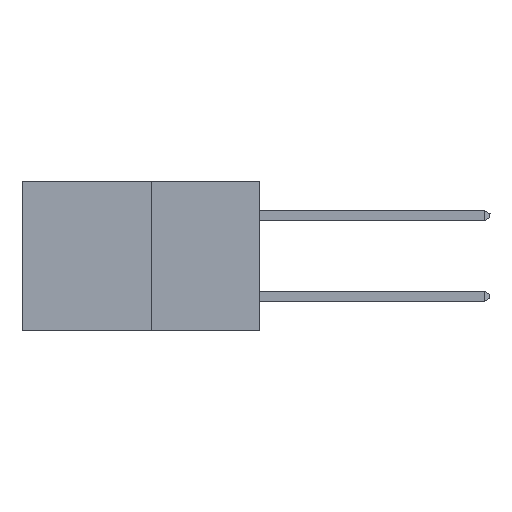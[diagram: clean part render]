
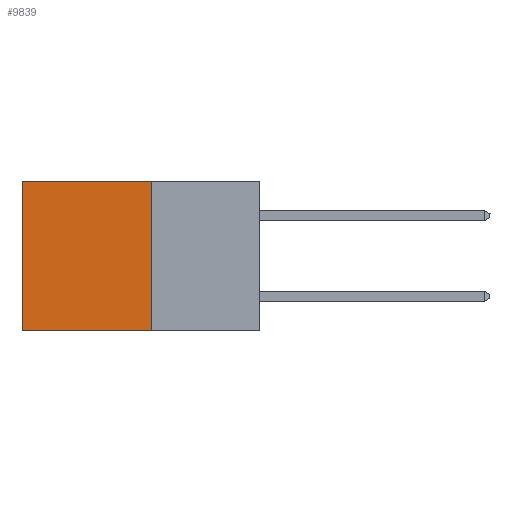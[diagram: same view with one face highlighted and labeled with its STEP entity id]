
A CAD part, left-side view. The second image highlights one B-rep face of the part: STEP entity #9839.
In plain terms, the highlighted planar face has unit normal (-1, 0, 0).
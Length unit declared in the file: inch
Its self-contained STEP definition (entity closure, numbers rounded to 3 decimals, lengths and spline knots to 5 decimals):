
#559 = VERTEX_POINT ( 'NONE', #7490 ) ;
#1075 = EDGE_CURVE ( 'NONE', #15030, #559, #17477, .T. ) ;
#1089 = VECTOR ( 'NONE', #19593, 39.37008 ) ;
#2191 = CARTESIAN_POINT ( 'NONE',  ( 0.277, 0.27, -0.37 ) ) ;
#3809 = DIRECTION ( 'NONE',  ( 0., 0., -1. ) ) ;
#5246 = ORIENTED_EDGE ( 'NONE', *, *, #15744, .T. ) ;
#5255 = DIRECTION ( 'NONE',  ( 0., 1., 0. ) ) ;
#5780 = DIRECTION ( 'NONE',  ( 0., 0., -1. ) ) ;
#6811 = LINE ( 'NONE', #18288, #15127 ) ;
#7490 = CARTESIAN_POINT ( 'NONE',  ( 0.277, 0.59, -0.37 ) ) ;
#9238 = EDGE_CURVE ( 'NONE', #15883, #559, #13239, .T. ) ;
#9664 = VECTOR ( 'NONE', #17323, 39.37008 ) ;
#9839 = ADVANCED_FACE ( 'NONE', ( #18073 ), #17810, .F. ) ;
#10019 = EDGE_CURVE ( 'NONE', #14950, #15030, #6811, .T. ) ;
#10610 = ORIENTED_EDGE ( 'NONE', *, *, #1075, .F. ) ;
#10669 = CARTESIAN_POINT ( 'NONE',  ( 0.277, 0.27, 0. ) ) ;
#11097 = ORIENTED_EDGE ( 'NONE', *, *, #10019, .F. ) ;
#11840 = ORIENTED_EDGE ( 'NONE', *, *, #9238, .T. ) ;
#13207 = DIRECTION ( 'NONE',  ( 1., 0., 0. ) ) ;
#13239 = LINE ( 'NONE', #18043, #1089 ) ;
#13891 = LINE ( 'NONE', #14625, #18014 ) ;
#13965 = CARTESIAN_POINT ( 'NONE',  ( 0.277, 0.27, -0.37 ) ) ;
#14625 = CARTESIAN_POINT ( 'NONE',  ( 0.277, 0.27, 0. ) ) ;
#14950 = VERTEX_POINT ( 'NONE', #10669 ) ;
#15030 = VERTEX_POINT ( 'NONE', #13965 ) ;
#15127 = VECTOR ( 'NONE', #5780, 39.37008 ) ;
#15744 = EDGE_CURVE ( 'NONE', #14950, #15883, #13891, .T. ) ;
#15883 = VERTEX_POINT ( 'NONE', #16467 ) ;
#16467 = CARTESIAN_POINT ( 'NONE',  ( 0.277, 0.59, 0. ) ) ;
#17307 = CARTESIAN_POINT ( 'NONE',  ( 0.277, 0.27, -0.37 ) ) ;
#17323 = DIRECTION ( 'NONE',  ( 0., 1., 0. ) ) ;
#17477 = LINE ( 'NONE', #17307, #9664 ) ;
#17810 = PLANE ( 'NONE',  #18441 ) ;
#18014 = VECTOR ( 'NONE', #5255, 39.37008 ) ;
#18043 = CARTESIAN_POINT ( 'NONE',  ( 0.277, 0.59, -0.37 ) ) ;
#18073 = FACE_OUTER_BOUND ( 'NONE', #19993, .T. ) ;
#18288 = CARTESIAN_POINT ( 'NONE',  ( 0.277, 0.27, -0.37 ) ) ;
#18441 = AXIS2_PLACEMENT_3D ( 'NONE', #2191, #13207, #3809 ) ;
#19593 = DIRECTION ( 'NONE',  ( 0., 0., -1. ) ) ;
#19993 = EDGE_LOOP ( 'NONE', ( #11840, #10610, #11097, #5246 ) ) ;
